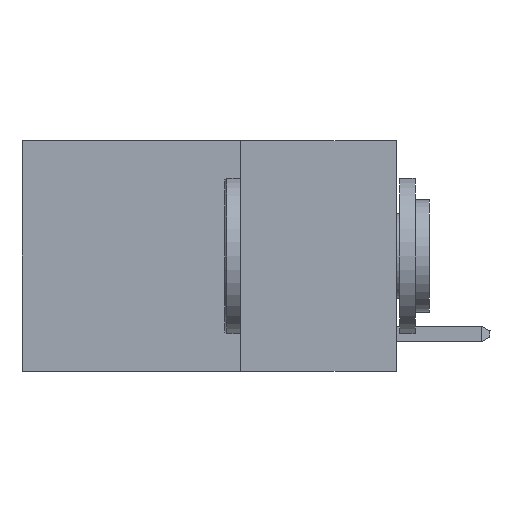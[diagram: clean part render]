
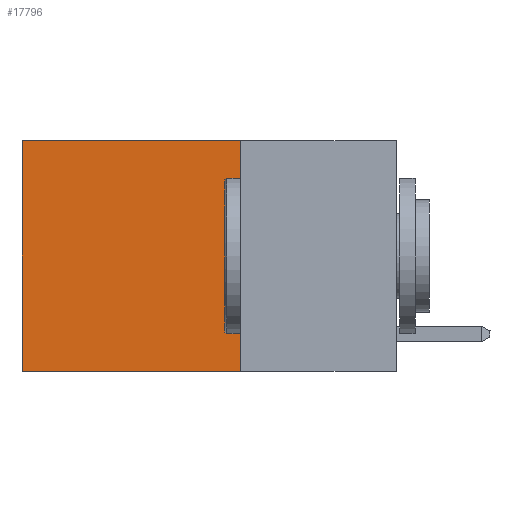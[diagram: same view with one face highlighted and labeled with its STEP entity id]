
A CAD part, left-side view. The second image highlights one B-rep face of the part: STEP entity #17796.
In plain terms, the highlighted planar face has unit normal (-1, 0, 0).
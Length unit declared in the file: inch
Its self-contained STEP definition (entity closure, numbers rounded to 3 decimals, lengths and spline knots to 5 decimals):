
#489 = VECTOR ( 'NONE', #21626, 39.37008 ) ;
#613 = VERTEX_POINT ( 'NONE', #6170 ) ;
#721 = EDGE_LOOP ( 'NONE', ( #11565, #12985, #11513, #6716 ) ) ;
#792 = LINE ( 'NONE', #9133, #3989 ) ;
#1297 = VECTOR ( 'NONE', #21843, 39.37008 ) ;
#2789 = VECTOR ( 'NONE', #17215, 39.37008 ) ;
#3989 = VECTOR ( 'NONE', #9506, 39.37008 ) ;
#4831 = EDGE_CURVE ( 'NONE', #8840, #15733, #792, .T. ) ;
#4976 = LINE ( 'NONE', #8177, #489 ) ;
#5021 = CARTESIAN_POINT ( 'NONE',  ( 0.2625, 0.6, 0. ) ) ;
#6170 = CARTESIAN_POINT ( 'NONE',  ( 0.2625, 0.25, -0.37 ) ) ;
#6461 = CARTESIAN_POINT ( 'NONE',  ( 0.2625, 0.25, 0. ) ) ;
#6716 = ORIENTED_EDGE ( 'NONE', *, *, #4831, .T. ) ;
#6767 = CARTESIAN_POINT ( 'NONE',  ( 0.2625, 0.6, 0. ) ) ;
#7541 = FACE_OUTER_BOUND ( 'NONE', #721, .T. ) ;
#8177 = CARTESIAN_POINT ( 'NONE',  ( 0.2625, 0.25, -0.37 ) ) ;
#8384 = EDGE_CURVE ( 'NONE', #8840, #613, #18125, .T. ) ;
#8840 = VERTEX_POINT ( 'NONE', #11479 ) ;
#9133 = CARTESIAN_POINT ( 'NONE',  ( 0.2625, 0.25, 0. ) ) ;
#9506 = DIRECTION ( 'NONE',  ( 0., 1., 0. ) ) ;
#10224 = AXIS2_PLACEMENT_3D ( 'NONE', #6461, #20030, #11822 ) ;
#11479 = CARTESIAN_POINT ( 'NONE',  ( 0.2625, 0.25, 0. ) ) ;
#11513 = ORIENTED_EDGE ( 'NONE', *, *, #8384, .F. ) ;
#11565 = ORIENTED_EDGE ( 'NONE', *, *, #12778, .T. ) ;
#11822 = DIRECTION ( 'NONE',  ( 0., 0., -1. ) ) ;
#11952 = LINE ( 'NONE', #6767, #1297 ) ;
#12162 = VERTEX_POINT ( 'NONE', #15264 ) ;
#12778 = EDGE_CURVE ( 'NONE', #15733, #12162, #11952, .T. ) ;
#12985 = ORIENTED_EDGE ( 'NONE', *, *, #21411, .F. ) ;
#15264 = CARTESIAN_POINT ( 'NONE',  ( 0.2625, 0.6, -0.37 ) ) ;
#15511 = CARTESIAN_POINT ( 'NONE',  ( 0.2625, 0.25, 0. ) ) ;
#15733 = VERTEX_POINT ( 'NONE', #5021 ) ;
#17215 = DIRECTION ( 'NONE',  ( 0., 0., -1. ) ) ;
#17796 = ADVANCED_FACE ( 'NONE', ( #7541 ), #21883, .F. ) ;
#18125 = LINE ( 'NONE', #15511, #2789 ) ;
#20030 = DIRECTION ( 'NONE',  ( 1., 0., 0. ) ) ;
#21411 = EDGE_CURVE ( 'NONE', #613, #12162, #4976, .T. ) ;
#21626 = DIRECTION ( 'NONE',  ( 0., 1., 0. ) ) ;
#21843 = DIRECTION ( 'NONE',  ( 0., 0., -1. ) ) ;
#21883 = PLANE ( 'NONE',  #10224 ) ;
